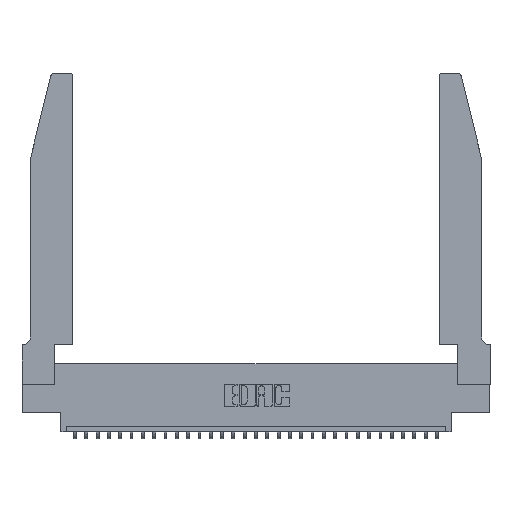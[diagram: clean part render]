
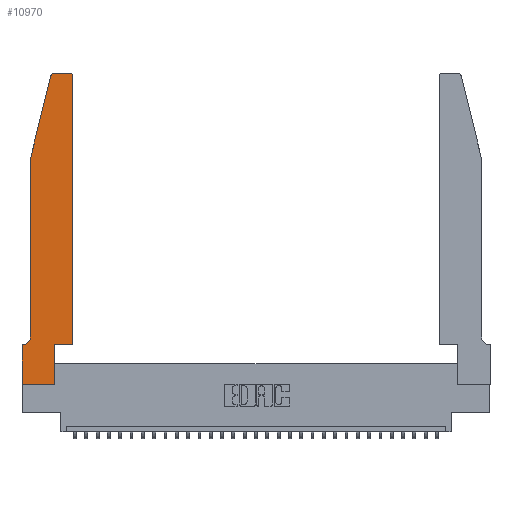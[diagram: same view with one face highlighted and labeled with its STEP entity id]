
A CAD part, top view. The second image highlights one B-rep face of the part: STEP entity #10970.
In plain terms, the highlighted planar face has unit normal (0, 0, 1).
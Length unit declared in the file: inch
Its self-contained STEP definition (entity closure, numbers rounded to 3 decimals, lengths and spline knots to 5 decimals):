
#5 = VECTOR ( 'NONE', #14011, 39.37008 ) ;
#516 = LINE ( 'NONE', #29657, #912 ) ;
#554 = VECTOR ( 'NONE', #11036, 39.37008 ) ;
#870 = DIRECTION ( 'NONE',  ( 0., 1., 0. ) ) ;
#912 = VECTOR ( 'NONE', #12771, 39.37008 ) ;
#916 = CARTESIAN_POINT ( 'NONE',  ( 0.0055, 0.35, 0.37 ) ) ;
#2289 = CARTESIAN_POINT ( 'NONE',  ( 0., 0., 0.37 ) ) ;
#2725 = CARTESIAN_POINT ( 'NONE',  ( 0., 0., 0.37 ) ) ;
#2890 = LINE ( 'NONE', #28786, #27940 ) ;
#3026 = VERTEX_POINT ( 'NONE', #14165 ) ;
#3225 = ORIENTED_EDGE ( 'NONE', *, *, #9616, .T. ) ;
#3905 = DIRECTION ( 'NONE',  ( 0., 1., 0. ) ) ;
#4107 = DIRECTION ( 'NONE',  ( -0.239, -0.971, 0. ) ) ;
#4555 = CARTESIAN_POINT ( 'NONE',  ( 0.4205, 2.72, 0.37 ) ) ;
#4743 = DIRECTION ( 'NONE',  ( 0., 0., 1. ) ) ;
#4759 = CIRCLE ( 'NONE', #28956, 0.03 ) ;
#4953 = VECTOR ( 'NONE', #21597, 39.37008 ) ;
#5597 = VERTEX_POINT ( 'NONE', #916 ) ;
#5692 = ORIENTED_EDGE ( 'NONE', *, *, #28671, .T. ) ;
#6205 = CARTESIAN_POINT ( 'NONE',  ( 0.0755, 0.42, 0.37 ) ) ;
#6214 = PLANE ( 'NONE',  #24276 ) ;
#6693 = VERTEX_POINT ( 'NONE', #11544 ) ;
#6921 = VERTEX_POINT ( 'NONE', #25334 ) ;
#7176 = CARTESIAN_POINT ( 'NONE',  ( 0.4205, 2.75, 0.37 ) ) ;
#7345 = DIRECTION ( 'NONE',  ( 0., 0., -1. ) ) ;
#7537 = VECTOR ( 'NONE', #870, 39.37008 ) ;
#7662 = ORIENTED_EDGE ( 'NONE', *, *, #29124, .T. ) ;
#8519 = CARTESIAN_POINT ( 'NONE',  ( 0., 0.35, 0.37 ) ) ;
#9015 = VERTEX_POINT ( 'NONE', #10690 ) ;
#9187 = LINE ( 'NONE', #15472, #554 ) ;
#9573 = LINE ( 'NONE', #24551, #29372 ) ;
#9576 = DIRECTION ( 'NONE',  ( 1., 0., 0. ) ) ;
#9616 = EDGE_CURVE ( 'NONE', #6693, #21924, #9187, .T. ) ;
#9668 = ORIENTED_EDGE ( 'NONE', *, *, #20889, .T. ) ;
#9831 = EDGE_CURVE ( 'NONE', #17893, #6693, #9573, .T. ) ;
#9954 = LINE ( 'NONE', #29917, #13621 ) ;
#10460 = CARTESIAN_POINT ( 'NONE',  ( 0., 0.35, 0.37 ) ) ;
#10501 = LINE ( 'NONE', #24681, #7537 ) ;
#10690 = CARTESIAN_POINT ( 'NONE',  ( 0.2865, 0., 0.37 ) ) ;
#10970 = ADVANCED_FACE ( 'NONE', ( #28198 ), #6214, .T. ) ;
#11005 = VERTEX_POINT ( 'NONE', #15864 ) ;
#11036 = DIRECTION ( 'NONE',  ( 0., -1., 0. ) ) ;
#11060 = LINE ( 'NONE', #24028, #18138 ) ;
#11255 = VERTEX_POINT ( 'NONE', #7176 ) ;
#11544 = CARTESIAN_POINT ( 'NONE',  ( 0.0755, 2., 0.37 ) ) ;
#12017 = VERTEX_POINT ( 'NONE', #10460 ) ;
#12055 = EDGE_CURVE ( 'NONE', #15603, #11005, #10501, .T. ) ;
#12287 = DIRECTION ( 'NONE',  ( 0., 0., 1. ) ) ;
#12491 = CARTESIAN_POINT ( 'NONE',  ( 0.284, 2.72, 0.37 ) ) ;
#12771 = DIRECTION ( 'NONE',  ( -1., 0., 0. ) ) ;
#13621 = VECTOR ( 'NONE', #3905, 39.37008 ) ;
#13715 = EDGE_CURVE ( 'NONE', #11005, #11255, #23502, .T. ) ;
#14011 = DIRECTION ( 'NONE',  ( 0., -1., 0. ) ) ;
#14076 = DIRECTION ( 'NONE',  ( 1., 0., 0. ) ) ;
#14165 = CARTESIAN_POINT ( 'NONE',  ( 0.284, 2.75, 0.37 ) ) ;
#14647 = AXIS2_PLACEMENT_3D ( 'NONE', #4555, #4743, #14076 ) ;
#14660 = DIRECTION ( 'NONE',  ( 1., 0., 0. ) ) ;
#14684 = EDGE_CURVE ( 'NONE', #3026, #17893, #4759, .T. ) ;
#15472 = CARTESIAN_POINT ( 'NONE',  ( 0.0755, 2., 0.37 ) ) ;
#15603 = VERTEX_POINT ( 'NONE', #25915 ) ;
#15864 = CARTESIAN_POINT ( 'NONE',  ( 0.4505, 2.72, 0.37 ) ) ;
#17335 = ORIENTED_EDGE ( 'NONE', *, *, #12055, .T. ) ;
#17551 = ORIENTED_EDGE ( 'NONE', *, *, #27543, .T. ) ;
#17621 = DIRECTION ( 'NONE',  ( -1., 0., 0. ) ) ;
#17893 = VERTEX_POINT ( 'NONE', #26717 ) ;
#18138 = VECTOR ( 'NONE', #17621, 39.37008 ) ;
#18516 = ORIENTED_EDGE ( 'NONE', *, *, #25298, .T. ) ;
#18656 = LINE ( 'NONE', #2289, #5 ) ;
#19105 = LINE ( 'NONE', #30971, #4953 ) ;
#20544 = ORIENTED_EDGE ( 'NONE', *, *, #14684, .T. ) ;
#20711 = EDGE_LOOP ( 'NONE', ( #21931, #20544, #30341, #3225, #5692, #17551, #9668, #27415, #18516, #7662, #17335, #22265 ) ) ;
#20889 = EDGE_CURVE ( 'NONE', #12017, #27331, #18656, .T. ) ;
#21597 = DIRECTION ( 'NONE',  ( 1., 0., 0. ) ) ;
#21924 = VERTEX_POINT ( 'NONE', #6205 ) ;
#21931 = ORIENTED_EDGE ( 'NONE', *, *, #25130, .T. ) ;
#22038 = CARTESIAN_POINT ( 'NONE',  ( 0.0055, 0.42, 0.37 ) ) ;
#22265 = ORIENTED_EDGE ( 'NONE', *, *, #13715, .T. ) ;
#23502 = CIRCLE ( 'NONE', #14647, 0.03 ) ;
#24028 = CARTESIAN_POINT ( 'NONE',  ( 0.2605, 2.75, 0.37 ) ) ;
#24276 = AXIS2_PLACEMENT_3D ( 'NONE', #8519, #25438, #27832 ) ;
#24414 = EDGE_CURVE ( 'NONE', #27331, #9015, #2890, .T. ) ;
#24551 = CARTESIAN_POINT ( 'NONE',  ( 0.0755, 2., 0.37 ) ) ;
#24681 = CARTESIAN_POINT ( 'NONE',  ( 0.4505, 0.35, 0.37 ) ) ;
#25130 = EDGE_CURVE ( 'NONE', #11255, #3026, #11060, .T. ) ;
#25298 = EDGE_CURVE ( 'NONE', #9015, #6921, #9954, .T. ) ;
#25334 = CARTESIAN_POINT ( 'NONE',  ( 0.2865, 0.35, 0.37 ) ) ;
#25438 = DIRECTION ( 'NONE',  ( 0., 0., 1. ) ) ;
#25915 = CARTESIAN_POINT ( 'NONE',  ( 0.4505, 0.35, 0.37 ) ) ;
#25924 = AXIS2_PLACEMENT_3D ( 'NONE', #22038, #7345, #28865 ) ;
#26717 = CARTESIAN_POINT ( 'NONE',  ( 0.25487, 2.72718, 0.37 ) ) ;
#27331 = VERTEX_POINT ( 'NONE', #2725 ) ;
#27415 = ORIENTED_EDGE ( 'NONE', *, *, #24414, .T. ) ;
#27543 = EDGE_CURVE ( 'NONE', #5597, #12017, #516, .T. ) ;
#27832 = DIRECTION ( 'NONE',  ( 1., 0., 0. ) ) ;
#27940 = VECTOR ( 'NONE', #9576, 39.37008 ) ;
#28198 = FACE_OUTER_BOUND ( 'NONE', #20711, .T. ) ;
#28498 = CIRCLE ( 'NONE', #25924, 0.07 ) ;
#28671 = EDGE_CURVE ( 'NONE', #21924, #5597, #28498, .T. ) ;
#28786 = CARTESIAN_POINT ( 'NONE',  ( 0., 0., 0.37 ) ) ;
#28865 = DIRECTION ( 'NONE',  ( -1., 0., 0. ) ) ;
#28956 = AXIS2_PLACEMENT_3D ( 'NONE', #12491, #12287, #14660 ) ;
#29124 = EDGE_CURVE ( 'NONE', #6921, #15603, #19105, .T. ) ;
#29372 = VECTOR ( 'NONE', #4107, 39.37008 ) ;
#29657 = CARTESIAN_POINT ( 'NONE',  ( 0.0755, 0.35, 0.37 ) ) ;
#29917 = CARTESIAN_POINT ( 'NONE',  ( 0.2865, 0.35, 0.37 ) ) ;
#30341 = ORIENTED_EDGE ( 'NONE', *, *, #9831, .T. ) ;
#30971 = CARTESIAN_POINT ( 'NONE',  ( 0.4505, 0.35, 0.37 ) ) ;
